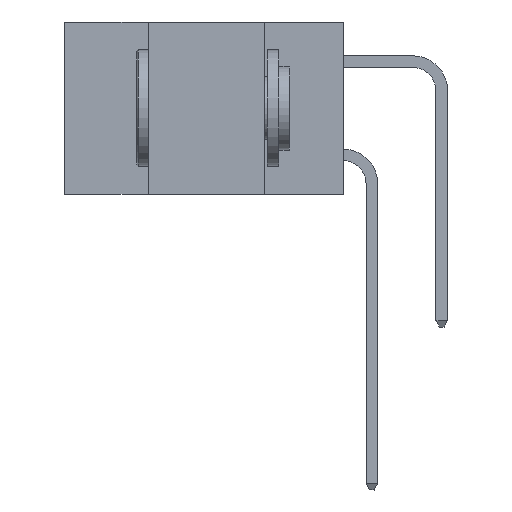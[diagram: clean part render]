
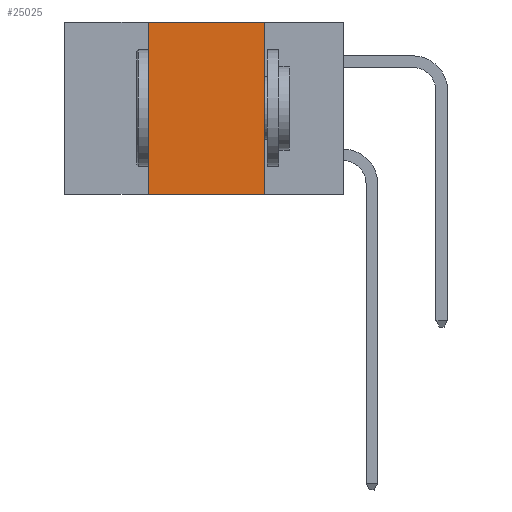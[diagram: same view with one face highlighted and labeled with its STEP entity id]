
A CAD part, left-side view. The second image highlights one B-rep face of the part: STEP entity #25025.
In plain terms, the highlighted planar face has unit normal (-1, 0, 0).
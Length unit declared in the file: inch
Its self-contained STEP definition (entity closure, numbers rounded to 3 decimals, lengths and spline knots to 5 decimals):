
#1492 = VERTEX_POINT ( 'NONE', #12369 ) ;
#1766 = EDGE_CURVE ( 'NONE', #13159, #1492, #29121, .T. ) ;
#1883 = VECTOR ( 'NONE', #28048, 39.37008 ) ;
#2927 = CARTESIAN_POINT ( 'NONE',  ( 0., 0.17, 0. ) ) ;
#6590 = EDGE_CURVE ( 'NONE', #18661, #13159, #31661, .T. ) ;
#10015 = VERTEX_POINT ( 'NONE', #10315 ) ;
#10043 = VECTOR ( 'NONE', #23990, 39.37008 ) ;
#10315 = CARTESIAN_POINT ( 'NONE',  ( 0., 0.17, -0.37 ) ) ;
#11306 = DIRECTION ( 'NONE',  ( 1., 0., 0. ) ) ;
#12130 = AXIS2_PLACEMENT_3D ( 'NONE', #16644, #11306, #30246 ) ;
#12365 = VECTOR ( 'NONE', #34222, 39.37008 ) ;
#12369 = CARTESIAN_POINT ( 'NONE',  ( 0., 0.17, 0. ) ) ;
#12616 = CARTESIAN_POINT ( 'NONE',  ( 0., 0.6, -0.37 ) ) ;
#13159 = VERTEX_POINT ( 'NONE', #14100 ) ;
#13220 = LINE ( 'NONE', #12616, #12365 ) ;
#13890 = ORIENTED_EDGE ( 'NONE', *, *, #32739, .F. ) ;
#14100 = CARTESIAN_POINT ( 'NONE',  ( 0., 0.42, 0. ) ) ;
#14482 = LINE ( 'NONE', #2927, #15343 ) ;
#15343 = VECTOR ( 'NONE', #21975, 39.37008 ) ;
#15764 = EDGE_CURVE ( 'NONE', #18661, #10015, #13220, .T. ) ;
#16472 = ORIENTED_EDGE ( 'NONE', *, *, #6590, .F. ) ;
#16644 = CARTESIAN_POINT ( 'NONE',  ( 0., 0.6, 0. ) ) ;
#17160 = EDGE_LOOP ( 'NONE', ( #13890, #34133, #16472, #24030 ) ) ;
#18661 = VERTEX_POINT ( 'NONE', #28723 ) ;
#21271 = CARTESIAN_POINT ( 'NONE',  ( 0., 0.42, 0. ) ) ;
#21975 = DIRECTION ( 'NONE',  ( 0., 0., -1. ) ) ;
#23990 = DIRECTION ( 'NONE',  ( 0., 0., 1. ) ) ;
#24030 = ORIENTED_EDGE ( 'NONE', *, *, #15764, .T. ) ;
#25025 = ADVANCED_FACE ( 'NONE', ( #30731 ), #27487, .F. ) ;
#26911 = CARTESIAN_POINT ( 'NONE',  ( 0., 0.6, 0. ) ) ;
#27487 = PLANE ( 'NONE',  #12130 ) ;
#28048 = DIRECTION ( 'NONE',  ( 0., -1., 0. ) ) ;
#28723 = CARTESIAN_POINT ( 'NONE',  ( 0., 0.42, -0.37 ) ) ;
#29121 = LINE ( 'NONE', #26911, #1883 ) ;
#30246 = DIRECTION ( 'NONE',  ( 0., 0., -1. ) ) ;
#30731 = FACE_OUTER_BOUND ( 'NONE', #17160, .T. ) ;
#31661 = LINE ( 'NONE', #21271, #10043 ) ;
#32739 = EDGE_CURVE ( 'NONE', #1492, #10015, #14482, .T. ) ;
#34133 = ORIENTED_EDGE ( 'NONE', *, *, #1766, .F. ) ;
#34222 = DIRECTION ( 'NONE',  ( 0., -1., 0. ) ) ;
